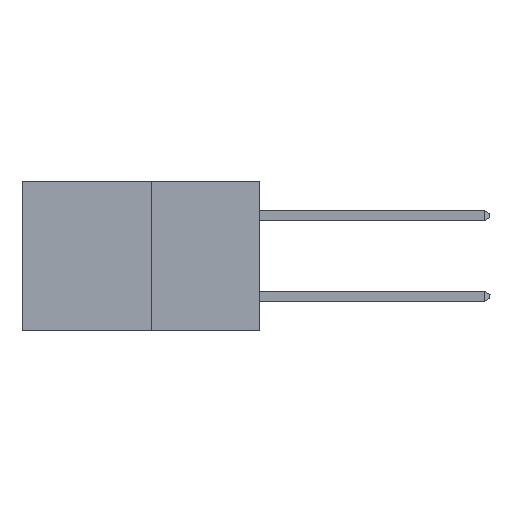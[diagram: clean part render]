
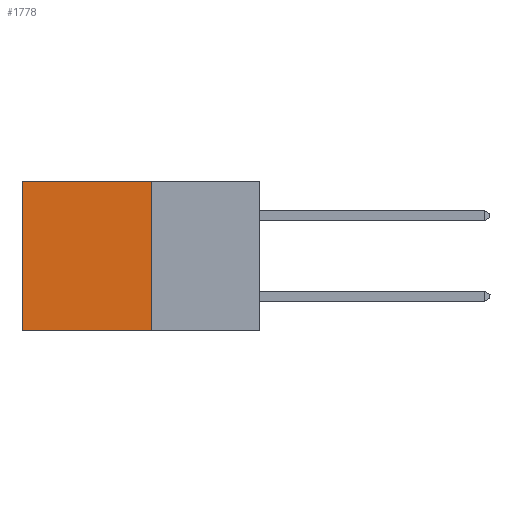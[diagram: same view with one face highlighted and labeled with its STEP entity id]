
A CAD part, left-side view. The second image highlights one B-rep face of the part: STEP entity #1778.
In plain terms, the highlighted planar face has unit normal (-1, 0, 0).
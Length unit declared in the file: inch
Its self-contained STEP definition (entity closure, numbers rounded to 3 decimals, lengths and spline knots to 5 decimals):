
#380 = LINE ( 'NONE', #5781, #3965 ) ;
#473 = ORIENTED_EDGE ( 'NONE', *, *, #7198, .F. ) ;
#499 = EDGE_LOOP ( 'NONE', ( #5235, #473, #8037, #10487 ) ) ;
#558 = PLANE ( 'NONE',  #7520 ) ;
#1778 = ADVANCED_FACE ( 'NONE', ( #6800 ), #558, .F. ) ;
#2555 = DIRECTION ( 'NONE',  ( 1., 0., 0. ) ) ;
#2822 = CARTESIAN_POINT ( 'NONE',  ( 0.277, 0.27, -0.37 ) ) ;
#3157 = DIRECTION ( 'NONE',  ( 0., 0., -1. ) ) ;
#3387 = DIRECTION ( 'NONE',  ( 0., 1., 0. ) ) ;
#3965 = VECTOR ( 'NONE', #11207, 39.37008 ) ;
#4053 = EDGE_CURVE ( 'NONE', #11650, #8867, #7554, .T. ) ;
#4242 = CARTESIAN_POINT ( 'NONE',  ( 0.277, 0.59, -0.37 ) ) ;
#4910 = VECTOR ( 'NONE', #10903, 39.37008 ) ;
#5023 = VECTOR ( 'NONE', #6298, 39.37008 ) ;
#5075 = VECTOR ( 'NONE', #3387, 39.37008 ) ;
#5195 = LINE ( 'NONE', #6245, #4910 ) ;
#5235 = ORIENTED_EDGE ( 'NONE', *, *, #6430, .T. ) ;
#5291 = CARTESIAN_POINT ( 'NONE',  ( 0.277, 0.27, 0. ) ) ;
#5781 = CARTESIAN_POINT ( 'NONE',  ( 0.277, 0.27, -0.37 ) ) ;
#6245 = CARTESIAN_POINT ( 'NONE',  ( 0.277, 0.27, -0.37 ) ) ;
#6298 = DIRECTION ( 'NONE',  ( 0., 0., -1. ) ) ;
#6430 = EDGE_CURVE ( 'NONE', #8867, #10905, #9939, .T. ) ;
#6657 = CARTESIAN_POINT ( 'NONE',  ( 0.277, 0.59, 0. ) ) ;
#6800 = FACE_OUTER_BOUND ( 'NONE', #499, .T. ) ;
#7198 = EDGE_CURVE ( 'NONE', #8432, #10905, #380, .T. ) ;
#7520 = AXIS2_PLACEMENT_3D ( 'NONE', #2822, #2555, #3157 ) ;
#7554 = LINE ( 'NONE', #5291, #5075 ) ;
#8037 = ORIENTED_EDGE ( 'NONE', *, *, #10960, .F. ) ;
#8432 = VERTEX_POINT ( 'NONE', #9111 ) ;
#8867 = VERTEX_POINT ( 'NONE', #6657 ) ;
#9055 = CARTESIAN_POINT ( 'NONE',  ( 0.277, 0.59, -0.37 ) ) ;
#9111 = CARTESIAN_POINT ( 'NONE',  ( 0.277, 0.27, -0.37 ) ) ;
#9882 = CARTESIAN_POINT ( 'NONE',  ( 0.277, 0.27, 0. ) ) ;
#9939 = LINE ( 'NONE', #4242, #5023 ) ;
#10487 = ORIENTED_EDGE ( 'NONE', *, *, #4053, .T. ) ;
#10903 = DIRECTION ( 'NONE',  ( 0., 0., -1. ) ) ;
#10905 = VERTEX_POINT ( 'NONE', #9055 ) ;
#10960 = EDGE_CURVE ( 'NONE', #11650, #8432, #5195, .T. ) ;
#11207 = DIRECTION ( 'NONE',  ( 0., 1., 0. ) ) ;
#11650 = VERTEX_POINT ( 'NONE', #9882 ) ;
